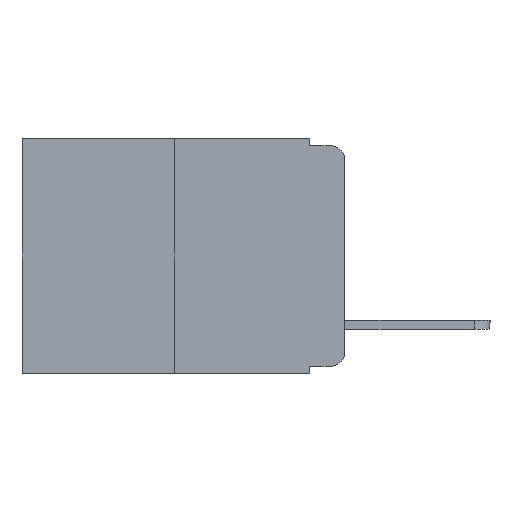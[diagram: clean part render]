
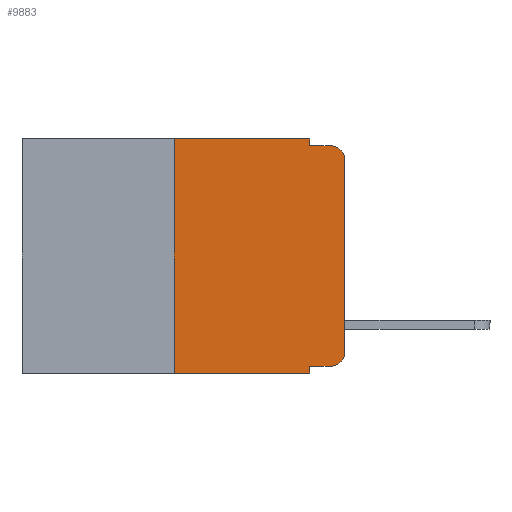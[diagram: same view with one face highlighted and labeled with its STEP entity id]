
A CAD part, left-side view. The second image highlights one B-rep face of the part: STEP entity #9883.
In plain terms, the highlighted planar face has unit normal (-1, 0, 0).
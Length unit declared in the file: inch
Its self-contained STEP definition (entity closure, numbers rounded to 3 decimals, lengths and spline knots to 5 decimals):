
#84 = ORIENTED_EDGE ( 'NONE', *, *, #10522, .T. ) ;
#179 = DIRECTION ( 'NONE',  ( 1., 0., 0. ) ) ;
#183 = CARTESIAN_POINT ( 'NONE',  ( 0., 0.051, 0. ) ) ;
#272 = DIRECTION ( 'NONE',  ( 0., 0., 1. ) ) ;
#482 = CARTESIAN_POINT ( 'NONE',  ( 0., 0.051, -0.01 ) ) ;
#658 = EDGE_CURVE ( 'NONE', #2429, #8291, #7915, .T. ) ;
#727 = DIRECTION ( 'NONE',  ( 0., 0., 1. ) ) ;
#1059 = VECTOR ( 'NONE', #727, 39.37008 ) ;
#1249 = CIRCLE ( 'NONE', #4086, 0.02 ) ;
#1613 = ORIENTED_EDGE ( 'NONE', *, *, #9380, .F. ) ;
#1808 = CARTESIAN_POINT ( 'NONE',  ( 0., 0.02, -0.313 ) ) ;
#1838 = CARTESIAN_POINT ( 'NONE',  ( 0., 0.02, -0.333 ) ) ;
#1867 = DIRECTION ( 'NONE',  ( 0., 0., -1. ) ) ;
#2018 = AXIS2_PLACEMENT_3D ( 'NONE', #5233, #7834, #10381 ) ;
#2037 = DIRECTION ( 'NONE',  ( -1., 0., 0. ) ) ;
#2170 = ORIENTED_EDGE ( 'NONE', *, *, #658, .T. ) ;
#2269 = VERTEX_POINT ( 'NONE', #10563 ) ;
#2429 = VERTEX_POINT ( 'NONE', #6966 ) ;
#2510 = VECTOR ( 'NONE', #10497, 39.37008 ) ;
#2562 = VERTEX_POINT ( 'NONE', #5673 ) ;
#2640 = VECTOR ( 'NONE', #10286, 39.37008 ) ;
#2665 = CARTESIAN_POINT ( 'NONE',  ( 0., 0.25, 0. ) ) ;
#2716 = EDGE_CURVE ( 'NONE', #3122, #5444, #5119, .T. ) ;
#3122 = VERTEX_POINT ( 'NONE', #183 ) ;
#3381 = ORIENTED_EDGE ( 'NONE', *, *, #6026, .T. ) ;
#3546 = VERTEX_POINT ( 'NONE', #10463 ) ;
#3862 = CARTESIAN_POINT ( 'NONE',  ( 0., 0.02, -0.01 ) ) ;
#4058 = LINE ( 'NONE', #8290, #7479 ) ;
#4086 = AXIS2_PLACEMENT_3D ( 'NONE', #1808, #2037, #1867 ) ;
#4281 = CARTESIAN_POINT ( 'NONE',  ( 0., 0.051, 0. ) ) ;
#4959 = DIRECTION ( 'NONE',  ( 0., 0., -1. ) ) ;
#5056 = VERTEX_POINT ( 'NONE', #3862 ) ;
#5119 = LINE ( 'NONE', #4281, #10966 ) ;
#5161 = DIRECTION ( 'NONE',  ( 0., 0., -1. ) ) ;
#5233 = CARTESIAN_POINT ( 'NONE',  ( 0., 0.02, -0.03 ) ) ;
#5272 = ORIENTED_EDGE ( 'NONE', *, *, #7286, .T. ) ;
#5410 = LINE ( 'NONE', #6011, #5691 ) ;
#5444 = VERTEX_POINT ( 'NONE', #482 ) ;
#5467 = CARTESIAN_POINT ( 'NONE',  ( 0., 0.051, -0.333 ) ) ;
#5495 = VECTOR ( 'NONE', #272, 39.37008 ) ;
#5673 = CARTESIAN_POINT ( 'NONE',  ( 0., 0.25, -0.343 ) ) ;
#5691 = VECTOR ( 'NONE', #10443, 39.37008 ) ;
#5834 = VECTOR ( 'NONE', #8911, 39.37008 ) ;
#5934 = CARTESIAN_POINT ( 'NONE',  ( 0., 0.473, 0. ) ) ;
#5952 = EDGE_CURVE ( 'NONE', #2562, #3546, #9354, .T. ) ;
#5985 = FACE_OUTER_BOUND ( 'NONE', #6840, .T. ) ;
#6011 = CARTESIAN_POINT ( 'NONE',  ( 0., 0.051, 0. ) ) ;
#6026 = EDGE_CURVE ( 'NONE', #2269, #8197, #8187, .T. ) ;
#6308 = EDGE_CURVE ( 'NONE', #2562, #10466, #6735, .T. ) ;
#6328 = CARTESIAN_POINT ( 'NONE',  ( 0., 0., -0.03 ) ) ;
#6735 = LINE ( 'NONE', #8347, #1059 ) ;
#6840 = EDGE_LOOP ( 'NONE', ( #2170, #84, #1613, #7690, #10649, #9570, #9406, #8161, #3381, #5272 ) ) ;
#6853 = CARTESIAN_POINT ( 'NONE',  ( 0., 0.473, -0.343 ) ) ;
#6927 = PLANE ( 'NONE',  #6953 ) ;
#6953 = AXIS2_PLACEMENT_3D ( 'NONE', #5934, #179, #5161 ) ;
#6966 = CARTESIAN_POINT ( 'NONE',  ( 0., 0., -0.313 ) ) ;
#7067 = LINE ( 'NONE', #7844, #2510 ) ;
#7286 = EDGE_CURVE ( 'NONE', #8197, #2429, #1249, .T. ) ;
#7479 = VECTOR ( 'NONE', #10815, 39.37008 ) ;
#7690 = ORIENTED_EDGE ( 'NONE', *, *, #2716, .F. ) ;
#7760 = EDGE_CURVE ( 'NONE', #10466, #3122, #7067, .T. ) ;
#7834 = DIRECTION ( 'NONE',  ( -1., 0., 0. ) ) ;
#7844 = CARTESIAN_POINT ( 'NONE',  ( 0., 0.473, 0. ) ) ;
#7915 = LINE ( 'NONE', #10567, #5495 ) ;
#8161 = ORIENTED_EDGE ( 'NONE', *, *, #9060, .F. ) ;
#8187 = LINE ( 'NONE', #5467, #5834 ) ;
#8197 = VERTEX_POINT ( 'NONE', #1838 ) ;
#8290 = CARTESIAN_POINT ( 'NONE',  ( 0., 0.051, -0.01 ) ) ;
#8291 = VERTEX_POINT ( 'NONE', #6328 ) ;
#8347 = CARTESIAN_POINT ( 'NONE',  ( 0., 0.25, 0. ) ) ;
#8911 = DIRECTION ( 'NONE',  ( 0., -1., 0. ) ) ;
#9060 = EDGE_CURVE ( 'NONE', #2269, #3546, #5410, .T. ) ;
#9354 = LINE ( 'NONE', #6853, #2640 ) ;
#9380 = EDGE_CURVE ( 'NONE', #5444, #5056, #4058, .T. ) ;
#9406 = ORIENTED_EDGE ( 'NONE', *, *, #5952, .T. ) ;
#9570 = ORIENTED_EDGE ( 'NONE', *, *, #6308, .F. ) ;
#9883 = ADVANCED_FACE ( 'NONE', ( #5985 ), #6927, .F. ) ;
#10286 = DIRECTION ( 'NONE',  ( 0., -1., 0. ) ) ;
#10381 = DIRECTION ( 'NONE',  ( 0., 0., -1. ) ) ;
#10443 = DIRECTION ( 'NONE',  ( 0., 0., -1. ) ) ;
#10463 = CARTESIAN_POINT ( 'NONE',  ( 0., 0.051, -0.343 ) ) ;
#10466 = VERTEX_POINT ( 'NONE', #2665 ) ;
#10497 = DIRECTION ( 'NONE',  ( 0., -1., 0. ) ) ;
#10522 = EDGE_CURVE ( 'NONE', #8291, #5056, #10723, .T. ) ;
#10563 = CARTESIAN_POINT ( 'NONE',  ( 0., 0.051, -0.333 ) ) ;
#10567 = CARTESIAN_POINT ( 'NONE',  ( 0., 0., 0. ) ) ;
#10649 = ORIENTED_EDGE ( 'NONE', *, *, #7760, .F. ) ;
#10723 = CIRCLE ( 'NONE', #2018, 0.02 ) ;
#10815 = DIRECTION ( 'NONE',  ( 0., -1., 0. ) ) ;
#10966 = VECTOR ( 'NONE', #4959, 39.37008 ) ;
